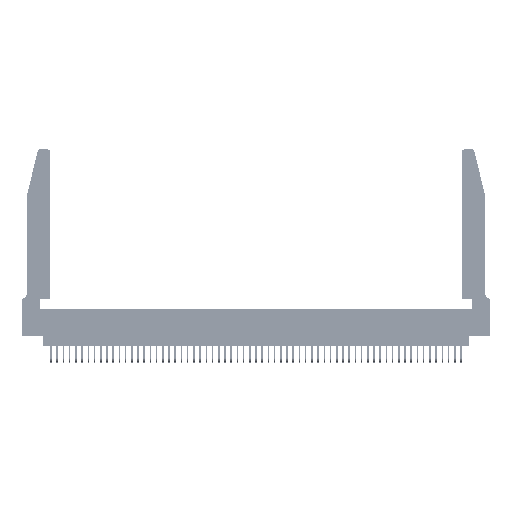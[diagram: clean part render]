
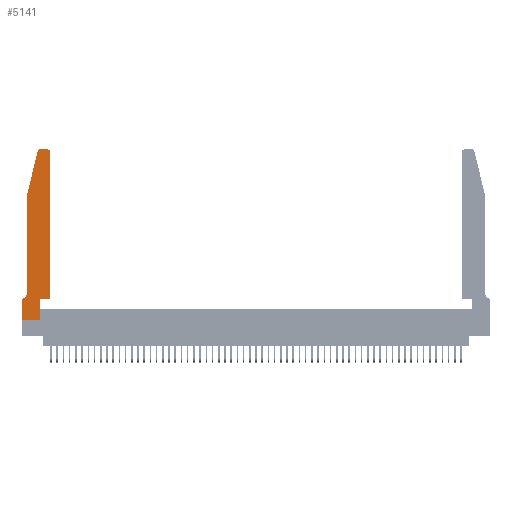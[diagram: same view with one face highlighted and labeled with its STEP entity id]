
A CAD part, top view. The second image highlights one B-rep face of the part: STEP entity #5141.
In plain terms, the highlighted planar face has unit normal (0, 0, 1).
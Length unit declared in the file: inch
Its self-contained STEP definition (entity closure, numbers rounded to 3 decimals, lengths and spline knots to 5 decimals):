
#104 = LINE ( 'NONE', #11121, #21724 ) ;
#289 = CARTESIAN_POINT ( 'NONE',  ( 0.2865, 0.35, 0.37 ) ) ;
#323 = DIRECTION ( 'NONE',  ( 1., 0., 0. ) ) ;
#427 = CARTESIAN_POINT ( 'NONE',  ( 0.0755, 0.35, 0.37 ) ) ;
#527 = CARTESIAN_POINT ( 'NONE',  ( 0.4505, 0.35, 0.37 ) ) ;
#528 = DIRECTION ( 'NONE',  ( -0.239, -0.971, 0. ) ) ;
#1064 = AXIS2_PLACEMENT_3D ( 'NONE', #30394, #43368, #17568 ) ;
#1228 = FACE_OUTER_BOUND ( 'NONE', #31310, .T. ) ;
#1887 = CARTESIAN_POINT ( 'NONE',  ( 0.0755, 2., 0.37 ) ) ;
#2056 = LINE ( 'NONE', #49496, #26370 ) ;
#3253 = CARTESIAN_POINT ( 'NONE',  ( 0., 0., 0.37 ) ) ;
#3585 = AXIS2_PLACEMENT_3D ( 'NONE', #22672, #52718, #26987 ) ;
#4763 = DIRECTION ( 'NONE',  ( -1., 0., 0. ) ) ;
#4915 = CARTESIAN_POINT ( 'NONE',  ( 0.4505, 0.35, 0.37 ) ) ;
#5141 = ADVANCED_FACE ( 'NONE', ( #1228 ), #13249, .T. ) ;
#6054 = CARTESIAN_POINT ( 'NONE',  ( 0., 0., 0.37 ) ) ;
#6298 = LINE ( 'NONE', #4915, #27881 ) ;
#7643 = LINE ( 'NONE', #36683, #16375 ) ;
#7870 = CARTESIAN_POINT ( 'NONE',  ( 0.4505, 0.35, 0.37 ) ) ;
#8008 = CIRCLE ( 'NONE', #3585, 0.07 ) ;
#8359 = LINE ( 'NONE', #3253, #18449 ) ;
#8804 = LINE ( 'NONE', #427, #40452 ) ;
#9091 = EDGE_CURVE ( 'NONE', #47697, #13304, #104, .T. ) ;
#9209 = DIRECTION ( 'NONE',  ( 0., 1., 0. ) ) ;
#11121 = CARTESIAN_POINT ( 'NONE',  ( 0.0755, 2., 0.37 ) ) ;
#11953 = DIRECTION ( 'NONE',  ( 1., 0., 0. ) ) ;
#13249 = PLANE ( 'NONE',  #1064 ) ;
#13304 = VERTEX_POINT ( 'NONE', #54704 ) ;
#13375 = ORIENTED_EDGE ( 'NONE', *, *, #9091, .T. ) ;
#13669 = AXIS2_PLACEMENT_3D ( 'NONE', #46439, #20674, #50736 ) ;
#16375 = VECTOR ( 'NONE', #41049, 39.37008 ) ;
#17439 = VECTOR ( 'NONE', #22042, 39.37008 ) ;
#17568 = DIRECTION ( 'NONE',  ( 1., 0., 0. ) ) ;
#18449 = VECTOR ( 'NONE', #11953, 39.37008 ) ;
#19049 = EDGE_CURVE ( 'NONE', #23319, #41711, #7643, .T. ) ;
#20674 = DIRECTION ( 'NONE',  ( 0., 0., 1. ) ) ;
#21225 = VERTEX_POINT ( 'NONE', #21481 ) ;
#21356 = EDGE_CURVE ( 'NONE', #46906, #25284, #45200, .T. ) ;
#21481 = CARTESIAN_POINT ( 'NONE',  ( 0.284, 2.75, 0.37 ) ) ;
#21724 = VECTOR ( 'NONE', #49854, 39.37008 ) ;
#22042 = DIRECTION ( 'NONE',  ( 1., 0., 0. ) ) ;
#22095 = ORIENTED_EDGE ( 'NONE', *, *, #19049, .T. ) ;
#22672 = CARTESIAN_POINT ( 'NONE',  ( 0.0055, 0.42, 0.37 ) ) ;
#23161 = ORIENTED_EDGE ( 'NONE', *, *, #29003, .T. ) ;
#23170 = ORIENTED_EDGE ( 'NONE', *, *, #52884, .T. ) ;
#23319 = VERTEX_POINT ( 'NONE', #46497 ) ;
#23428 = ORIENTED_EDGE ( 'NONE', *, *, #45192, .T. ) ;
#25284 = VERTEX_POINT ( 'NONE', #289 ) ;
#26177 = VERTEX_POINT ( 'NONE', #32229 ) ;
#26206 = ORIENTED_EDGE ( 'NONE', *, *, #46139, .T. ) ;
#26207 = DIRECTION ( 'NONE',  ( 0., 0., 1. ) ) ;
#26370 = VECTOR ( 'NONE', #53838, 39.37008 ) ;
#26987 = DIRECTION ( 'NONE',  ( -1., 0., 0. ) ) ;
#27881 = VECTOR ( 'NONE', #30747, 39.37008 ) ;
#28499 = VERTEX_POINT ( 'NONE', #32085 ) ;
#28728 = EDGE_CURVE ( 'NONE', #41711, #46906, #8359, .T. ) ;
#29003 = EDGE_CURVE ( 'NONE', #42492, #26177, #6298, .T. ) ;
#29100 = LINE ( 'NONE', #52307, #30444 ) ;
#30394 = CARTESIAN_POINT ( 'NONE',  ( 0., 0.35, 0.37 ) ) ;
#30444 = VECTOR ( 'NONE', #528, 39.37008 ) ;
#30747 = DIRECTION ( 'NONE',  ( 0., 1., 0. ) ) ;
#31110 = ORIENTED_EDGE ( 'NONE', *, *, #21356, .T. ) ;
#31310 = EDGE_LOOP ( 'NONE', ( #53199, #26206, #44146, #13375, #46267, #23428, #22095, #46828, #31110, #43516, #23161, #23170 ) ) ;
#32085 = CARTESIAN_POINT ( 'NONE',  ( 0.4205, 2.75, 0.37 ) ) ;
#32229 = CARTESIAN_POINT ( 'NONE',  ( 0.4505, 2.72, 0.37 ) ) ;
#33364 = EDGE_CURVE ( 'NONE', #28499, #21225, #2056, .T. ) ;
#34966 = CARTESIAN_POINT ( 'NONE',  ( 0.2865, 0.35, 0.37 ) ) ;
#35088 = CARTESIAN_POINT ( 'NONE',  ( 0.2865, 0., 0.37 ) ) ;
#36683 = CARTESIAN_POINT ( 'NONE',  ( 0., 0., 0.37 ) ) ;
#37087 = CIRCLE ( 'NONE', #13669, 0.03 ) ;
#37903 = CARTESIAN_POINT ( 'NONE',  ( 0.0055, 0.35, 0.37 ) ) ;
#40117 = EDGE_CURVE ( 'NONE', #48449, #47697, #29100, .T. ) ;
#40452 = VECTOR ( 'NONE', #4763, 39.37008 ) ;
#41049 = DIRECTION ( 'NONE',  ( 0., -1., 0. ) ) ;
#41160 = CARTESIAN_POINT ( 'NONE',  ( 0.25487, 2.72718, 0.37 ) ) ;
#41705 = LINE ( 'NONE', #527, #17439 ) ;
#41711 = VERTEX_POINT ( 'NONE', #6054 ) ;
#42492 = VERTEX_POINT ( 'NONE', #7870 ) ;
#43368 = DIRECTION ( 'NONE',  ( 0., 0., 1. ) ) ;
#43516 = ORIENTED_EDGE ( 'NONE', *, *, #46196, .T. ) ;
#44146 = ORIENTED_EDGE ( 'NONE', *, *, #40117, .T. ) ;
#44982 = AXIS2_PLACEMENT_3D ( 'NONE', #51917, #26207, #323 ) ;
#45009 = VERTEX_POINT ( 'NONE', #37903 ) ;
#45192 = EDGE_CURVE ( 'NONE', #45009, #23319, #8804, .T. ) ;
#45200 = LINE ( 'NONE', #34966, #55273 ) ;
#46139 = EDGE_CURVE ( 'NONE', #21225, #48449, #53136, .T. ) ;
#46196 = EDGE_CURVE ( 'NONE', #25284, #42492, #41705, .T. ) ;
#46267 = ORIENTED_EDGE ( 'NONE', *, *, #54205, .T. ) ;
#46439 = CARTESIAN_POINT ( 'NONE',  ( 0.4205, 2.72, 0.37 ) ) ;
#46497 = CARTESIAN_POINT ( 'NONE',  ( 0., 0.35, 0.37 ) ) ;
#46828 = ORIENTED_EDGE ( 'NONE', *, *, #28728, .T. ) ;
#46906 = VERTEX_POINT ( 'NONE', #35088 ) ;
#47697 = VERTEX_POINT ( 'NONE', #1887 ) ;
#48449 = VERTEX_POINT ( 'NONE', #41160 ) ;
#49496 = CARTESIAN_POINT ( 'NONE',  ( 0.2605, 2.75, 0.37 ) ) ;
#49854 = DIRECTION ( 'NONE',  ( 0., -1., 0. ) ) ;
#50736 = DIRECTION ( 'NONE',  ( 1., 0., 0. ) ) ;
#51917 = CARTESIAN_POINT ( 'NONE',  ( 0.284, 2.72, 0.37 ) ) ;
#52307 = CARTESIAN_POINT ( 'NONE',  ( 0.0755, 2., 0.37 ) ) ;
#52718 = DIRECTION ( 'NONE',  ( 0., 0., -1. ) ) ;
#52884 = EDGE_CURVE ( 'NONE', #26177, #28499, #37087, .T. ) ;
#53136 = CIRCLE ( 'NONE', #44982, 0.03 ) ;
#53199 = ORIENTED_EDGE ( 'NONE', *, *, #33364, .T. ) ;
#53838 = DIRECTION ( 'NONE',  ( -1., 0., 0. ) ) ;
#54205 = EDGE_CURVE ( 'NONE', #13304, #45009, #8008, .T. ) ;
#54704 = CARTESIAN_POINT ( 'NONE',  ( 0.0755, 0.42, 0.37 ) ) ;
#55273 = VECTOR ( 'NONE', #9209, 39.37008 ) ;
